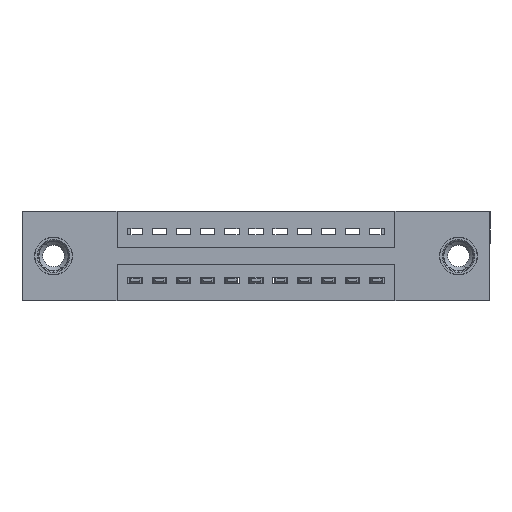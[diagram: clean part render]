
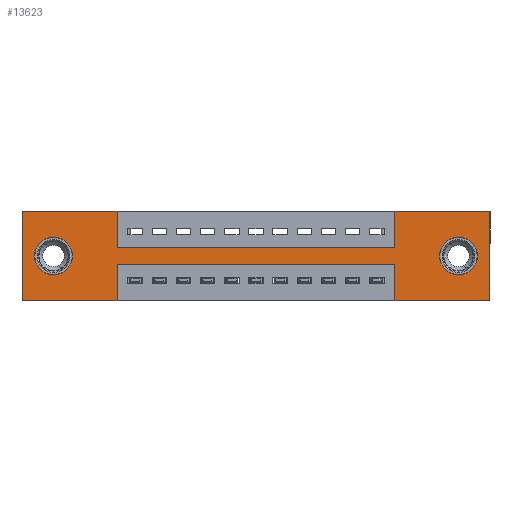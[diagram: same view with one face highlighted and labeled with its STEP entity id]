
A CAD part, front view. The second image highlights one B-rep face of the part: STEP entity #13623.
In plain terms, the highlighted planar face has unit normal (0, -1, 0).
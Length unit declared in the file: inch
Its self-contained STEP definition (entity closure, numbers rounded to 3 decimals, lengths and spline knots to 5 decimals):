
#2 = EDGE_CURVE ( 'NONE', #5333, #4402, #9368, .T. ) ;
#139 = DIRECTION ( 'NONE',  ( 0., 1., 0. ) ) ;
#191 = ORIENTED_EDGE ( 'NONE', *, *, #1973, .F. ) ;
#398 = CARTESIAN_POINT ( 'NONE',  ( 0., 0., -0.37 ) ) ;
#485 = EDGE_CURVE ( 'NONE', #795, #2446, #4529, .T. ) ;
#506 = DIRECTION ( 'NONE',  ( 0., 0., -1. ) ) ;
#595 = ORIENTED_EDGE ( 'NONE', *, *, #5292, .T. ) ;
#654 = ORIENTED_EDGE ( 'NONE', *, *, #12768, .F. ) ;
#729 = EDGE_CURVE ( 'NONE', #1405, #12767, #8587, .T. ) ;
#795 = VERTEX_POINT ( 'NONE', #8210 ) ;
#847 = DIRECTION ( 'NONE',  ( 0., 0., 1. ) ) ;
#877 = DIRECTION ( 'NONE',  ( 0., 0., -1. ) ) ;
#1405 = VERTEX_POINT ( 'NONE', #9074 ) ;
#1644 = CIRCLE ( 'NONE', #13799, 0.078 ) ;
#1798 = VECTOR ( 'NONE', #13404, 39.37008 ) ;
#1973 = EDGE_CURVE ( 'NONE', #2819, #11715, #7324, .T. ) ;
#2265 = ORIENTED_EDGE ( 'NONE', *, *, #13733, .F. ) ;
#2321 = VERTEX_POINT ( 'NONE', #9784 ) ;
#2352 = DIRECTION ( 'NONE',  ( 1., 0., 0. ) ) ;
#2419 = DIRECTION ( 'NONE',  ( 1., 0., 0. ) ) ;
#2435 = AXIS2_PLACEMENT_3D ( 'NONE', #14433, #5490, #3194 ) ;
#2446 = VERTEX_POINT ( 'NONE', #13654 ) ;
#2650 = PLANE ( 'NONE',  #12824 ) ;
#2798 = DIRECTION ( 'NONE',  ( 0., 0., 1. ) ) ;
#2819 = VERTEX_POINT ( 'NONE', #5190 ) ;
#2901 = VERTEX_POINT ( 'NONE', #5356 ) ;
#3194 = DIRECTION ( 'NONE',  ( 0., 0., 1. ) ) ;
#3637 = CARTESIAN_POINT ( 'NONE',  ( 1.935, 0., 0. ) ) ;
#3681 = FACE_BOUND ( 'NONE', #12311, .T. ) ;
#3814 = LINE ( 'NONE', #13303, #8981 ) ;
#3859 = DIRECTION ( 'NONE',  ( 0., 0., 1. ) ) ;
#3947 = DIRECTION ( 'NONE',  ( -1., 0., 0. ) ) ;
#4001 = LINE ( 'NONE', #7433, #7617 ) ;
#4161 = CARTESIAN_POINT ( 'NONE',  ( 0., 0., 0. ) ) ;
#4191 = ORIENTED_EDGE ( 'NONE', *, *, #4408, .F. ) ;
#4336 = VECTOR ( 'NONE', #3947, 39.37008 ) ;
#4402 = VERTEX_POINT ( 'NONE', #12759 ) ;
#4408 = EDGE_CURVE ( 'NONE', #5579, #7089, #13364, .T. ) ;
#4461 = CARTESIAN_POINT ( 'NONE',  ( 0., 0., 0. ) ) ;
#4492 = LINE ( 'NONE', #12032, #12998 ) ;
#4529 = LINE ( 'NONE', #8432, #5742 ) ;
#4916 = CARTESIAN_POINT ( 'NONE',  ( 0.13, 0., -0.263 ) ) ;
#5101 = LINE ( 'NONE', #4161, #7827 ) ;
#5156 = LINE ( 'NONE', #7350, #7658 ) ;
#5190 = CARTESIAN_POINT ( 'NONE',  ( 1.5425, 0., 0. ) ) ;
#5243 = CARTESIAN_POINT ( 'NONE',  ( 0., 0., 0. ) ) ;
#5281 = ORIENTED_EDGE ( 'NONE', *, *, #11863, .F. ) ;
#5292 = EDGE_CURVE ( 'NONE', #12767, #1405, #1644, .T. ) ;
#5333 = VERTEX_POINT ( 'NONE', #5243 ) ;
#5356 = CARTESIAN_POINT ( 'NONE',  ( 1.5425, 0., -0.22 ) ) ;
#5408 = CARTESIAN_POINT ( 'NONE',  ( 1.5425, 0., 0. ) ) ;
#5434 = VECTOR ( 'NONE', #12079, 39.37008 ) ;
#5490 = DIRECTION ( 'NONE',  ( 0., 1., 0. ) ) ;
#5579 = VERTEX_POINT ( 'NONE', #13415 ) ;
#5585 = VECTOR ( 'NONE', #2419, 39.37008 ) ;
#5597 = ORIENTED_EDGE ( 'NONE', *, *, #485, .F. ) ;
#5640 = ORIENTED_EDGE ( 'NONE', *, *, #13531, .T. ) ;
#5742 = VECTOR ( 'NONE', #10686, 39.37008 ) ;
#5817 = CARTESIAN_POINT ( 'NONE',  ( 0.3925, 0., -0.15 ) ) ;
#5963 = ORIENTED_EDGE ( 'NONE', *, *, #8299, .F. ) ;
#6148 = EDGE_LOOP ( 'NONE', ( #5597, #12541, #5281, #4191, #12912, #191, #5963, #2265, #654, #8172, #14288, #11154 ) ) ;
#6666 = CARTESIAN_POINT ( 'NONE',  ( 1.5425, 0., -0.37 ) ) ;
#6762 = VERTEX_POINT ( 'NONE', #4916 ) ;
#6816 = CIRCLE ( 'NONE', #7321, 0.078 ) ;
#7089 = VERTEX_POINT ( 'NONE', #6666 ) ;
#7172 = DIRECTION ( 'NONE',  ( 0., -1., 0. ) ) ;
#7321 = AXIS2_PLACEMENT_3D ( 'NONE', #8231, #11599, #3859 ) ;
#7324 = LINE ( 'NONE', #4461, #9223 ) ;
#7350 = CARTESIAN_POINT ( 'NONE',  ( 0., 0., -0.37 ) ) ;
#7399 = CARTESIAN_POINT ( 'NONE',  ( 0., 0., -0.37 ) ) ;
#7433 = CARTESIAN_POINT ( 'NONE',  ( 1.935, 0., 0. ) ) ;
#7578 = CARTESIAN_POINT ( 'NONE',  ( 0.13, 0., -0.107 ) ) ;
#7607 = ORIENTED_EDGE ( 'NONE', *, *, #729, .T. ) ;
#7617 = VECTOR ( 'NONE', #12783, 39.37008 ) ;
#7658 = VECTOR ( 'NONE', #8425, 39.37008 ) ;
#7827 = VECTOR ( 'NONE', #2798, 39.37008 ) ;
#8156 = EDGE_CURVE ( 'NONE', #2901, #795, #9075, .T. ) ;
#8172 = ORIENTED_EDGE ( 'NONE', *, *, #2, .F. ) ;
#8210 = CARTESIAN_POINT ( 'NONE',  ( 0.3925, 0., -0.22 ) ) ;
#8223 = CARTESIAN_POINT ( 'NONE',  ( 1.5425, 0., -0.15 ) ) ;
#8231 = CARTESIAN_POINT ( 'NONE',  ( 0.13, 0., -0.185 ) ) ;
#8299 = EDGE_CURVE ( 'NONE', #12636, #2819, #12380, .T. ) ;
#8425 = DIRECTION ( 'NONE',  ( -1., 0., 0. ) ) ;
#8432 = CARTESIAN_POINT ( 'NONE',  ( 0.3925, 0., -0.37 ) ) ;
#8587 = CIRCLE ( 'NONE', #10113, 0.078 ) ;
#8617 = CARTESIAN_POINT ( 'NONE',  ( 1.805, 0., -0.263 ) ) ;
#8716 = FACE_OUTER_BOUND ( 'NONE', #6148, .T. ) ;
#8749 = VECTOR ( 'NONE', #847, 39.37008 ) ;
#8824 = EDGE_CURVE ( 'NONE', #2321, #5333, #5101, .T. ) ;
#8981 = VECTOR ( 'NONE', #12418, 39.37008 ) ;
#9074 = CARTESIAN_POINT ( 'NONE',  ( 1.805, 0., -0.107 ) ) ;
#9075 = LINE ( 'NONE', #12036, #1798 ) ;
#9171 = CARTESIAN_POINT ( 'NONE',  ( 0., 0., 0. ) ) ;
#9223 = VECTOR ( 'NONE', #2352, 39.37008 ) ;
#9226 = CARTESIAN_POINT ( 'NONE',  ( 1.805, 0., -0.185 ) ) ;
#9350 = DIRECTION ( 'NONE',  ( 0., 0., -1. ) ) ;
#9368 = LINE ( 'NONE', #9171, #5585 ) ;
#9415 = ORIENTED_EDGE ( 'NONE', *, *, #9776, .T. ) ;
#9685 = DIRECTION ( 'NONE',  ( 0., 1., 0. ) ) ;
#9776 = EDGE_CURVE ( 'NONE', #12727, #6762, #11835, .T. ) ;
#9784 = CARTESIAN_POINT ( 'NONE',  ( 0., 0., -0.37 ) ) ;
#9956 = VERTEX_POINT ( 'NONE', #5817 ) ;
#10113 = AXIS2_PLACEMENT_3D ( 'NONE', #13506, #139, #13595 ) ;
#10686 = DIRECTION ( 'NONE',  ( 0., 0., -1. ) ) ;
#10981 = CARTESIAN_POINT ( 'NONE',  ( 0.3925, 0., -0.15 ) ) ;
#11042 = EDGE_CURVE ( 'NONE', #11715, #5579, #4001, .T. ) ;
#11154 = ORIENTED_EDGE ( 'NONE', *, *, #13329, .F. ) ;
#11599 = DIRECTION ( 'NONE',  ( 0., 1., 0. ) ) ;
#11677 = LINE ( 'NONE', #10981, #5434 ) ;
#11715 = VERTEX_POINT ( 'NONE', #3637 ) ;
#11835 = CIRCLE ( 'NONE', #2435, 0.078 ) ;
#11863 = EDGE_CURVE ( 'NONE', #7089, #2901, #3814, .T. ) ;
#12032 = CARTESIAN_POINT ( 'NONE',  ( 0.3925, 0., 0. ) ) ;
#12036 = CARTESIAN_POINT ( 'NONE',  ( 0.3925, 0., -0.22 ) ) ;
#12079 = DIRECTION ( 'NONE',  ( 1., 0., 0. ) ) ;
#12185 = FACE_BOUND ( 'NONE', #13580, .T. ) ;
#12311 = EDGE_LOOP ( 'NONE', ( #7607, #595 ) ) ;
#12380 = LINE ( 'NONE', #5408, #8749 ) ;
#12418 = DIRECTION ( 'NONE',  ( 0., 0., 1. ) ) ;
#12541 = ORIENTED_EDGE ( 'NONE', *, *, #8156, .F. ) ;
#12636 = VERTEX_POINT ( 'NONE', #8223 ) ;
#12727 = VERTEX_POINT ( 'NONE', #7578 ) ;
#12759 = CARTESIAN_POINT ( 'NONE',  ( 0.3925, 0., 0. ) ) ;
#12767 = VERTEX_POINT ( 'NONE', #8617 ) ;
#12768 = EDGE_CURVE ( 'NONE', #4402, #9956, #4492, .T. ) ;
#12783 = DIRECTION ( 'NONE',  ( 0., 0., -1. ) ) ;
#12824 = AXIS2_PLACEMENT_3D ( 'NONE', #398, #7172, #506 ) ;
#12912 = ORIENTED_EDGE ( 'NONE', *, *, #11042, .F. ) ;
#12998 = VECTOR ( 'NONE', #877, 39.37008 ) ;
#13303 = CARTESIAN_POINT ( 'NONE',  ( 1.5425, 0., -0.37 ) ) ;
#13329 = EDGE_CURVE ( 'NONE', #2446, #2321, #5156, .T. ) ;
#13364 = LINE ( 'NONE', #7399, #4336 ) ;
#13404 = DIRECTION ( 'NONE',  ( -1., 0., 0. ) ) ;
#13415 = CARTESIAN_POINT ( 'NONE',  ( 1.935, 0., -0.37 ) ) ;
#13506 = CARTESIAN_POINT ( 'NONE',  ( 1.805, 0., -0.185 ) ) ;
#13531 = EDGE_CURVE ( 'NONE', #6762, #12727, #6816, .T. ) ;
#13580 = EDGE_LOOP ( 'NONE', ( #9415, #5640 ) ) ;
#13595 = DIRECTION ( 'NONE',  ( 0., 0., -1. ) ) ;
#13623 = ADVANCED_FACE ( 'NONE', ( #3681, #12185, #8716 ), #2650, .T. ) ;
#13654 = CARTESIAN_POINT ( 'NONE',  ( 0.3925, 0., -0.37 ) ) ;
#13733 = EDGE_CURVE ( 'NONE', #9956, #12636, #11677, .T. ) ;
#13799 = AXIS2_PLACEMENT_3D ( 'NONE', #9226, #9685, #9350 ) ;
#14288 = ORIENTED_EDGE ( 'NONE', *, *, #8824, .F. ) ;
#14433 = CARTESIAN_POINT ( 'NONE',  ( 0.13, 0., -0.185 ) ) ;
